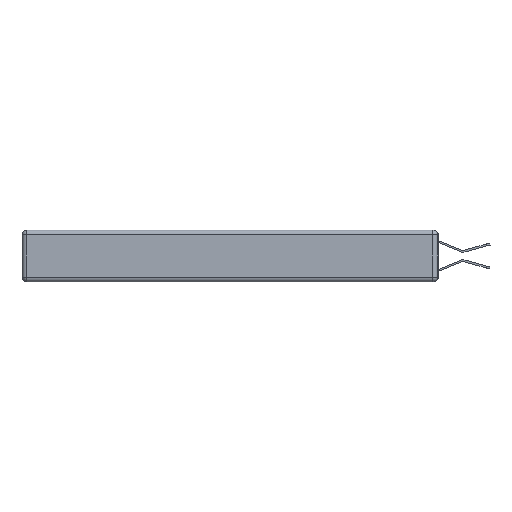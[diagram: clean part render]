
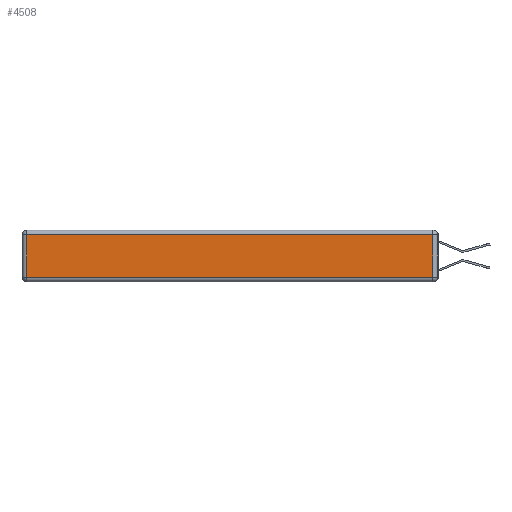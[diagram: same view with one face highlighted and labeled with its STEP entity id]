
A CAD part, left-side view. The second image highlights one B-rep face of the part: STEP entity #4508.
In plain terms, the highlighted planar face has unit normal (-1, 0, 0).
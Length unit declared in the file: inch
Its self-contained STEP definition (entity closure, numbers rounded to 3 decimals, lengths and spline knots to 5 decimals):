
#93 = DIRECTION ( 'NONE',  ( -1., 0., 0. ) ) ;
#626 = AXIS2_PLACEMENT_3D ( 'NONE', #4686, #93, #10742 ) ;
#983 = VECTOR ( 'NONE', #1084, 39.37008 ) ;
#1084 = DIRECTION ( 'NONE',  ( 0., 0., 1. ) ) ;
#1386 = CARTESIAN_POINT ( 'NONE',  ( 0., 2.72, -0.03 ) ) ;
#1850 = ORIENTED_EDGE ( 'NONE', *, *, #13331, .T. ) ;
#2027 = DIRECTION ( 'NONE',  ( 0., -1., 0. ) ) ;
#4492 = CARTESIAN_POINT ( 'NONE',  ( 0., 0., -0.313 ) ) ;
#4508 = ADVANCED_FACE ( 'NONE', ( #4921 ), #4766, .T. ) ;
#4585 = LINE ( 'NONE', #10493, #5303 ) ;
#4686 = CARTESIAN_POINT ( 'NONE',  ( 0., 0., -0.343 ) ) ;
#4766 = PLANE ( 'NONE',  #626 ) ;
#4921 = FACE_OUTER_BOUND ( 'NONE', #10962, .T. ) ;
#5303 = VECTOR ( 'NONE', #11910, 39.37008 ) ;
#7315 = CARTESIAN_POINT ( 'NONE',  ( 0., 0.03, -0.313 ) ) ;
#7919 = EDGE_CURVE ( 'NONE', #13001, #8813, #8820, .T. ) ;
#8742 = CARTESIAN_POINT ( 'NONE',  ( 0., 2.72, -0.313 ) ) ;
#8813 = VERTEX_POINT ( 'NONE', #1386 ) ;
#8820 = LINE ( 'NONE', #15041, #11105 ) ;
#9033 = VERTEX_POINT ( 'NONE', #8742 ) ;
#9103 = ORIENTED_EDGE ( 'NONE', *, *, #13421, .T. ) ;
#9520 = LINE ( 'NONE', #11983, #983 ) ;
#10493 = CARTESIAN_POINT ( 'NONE',  ( 0., 2.72, -0.343 ) ) ;
#10742 = DIRECTION ( 'NONE',  ( 0., 0., 1. ) ) ;
#10753 = ORIENTED_EDGE ( 'NONE', *, *, #13826, .T. ) ;
#10962 = EDGE_LOOP ( 'NONE', ( #10753, #9103, #13102, #1850 ) ) ;
#11105 = VECTOR ( 'NONE', #14879, 39.37008 ) ;
#11910 = DIRECTION ( 'NONE',  ( 0., 0., -1. ) ) ;
#11983 = CARTESIAN_POINT ( 'NONE',  ( 0., 0.03, -0.343 ) ) ;
#13001 = VERTEX_POINT ( 'NONE', #13452 ) ;
#13102 = ORIENTED_EDGE ( 'NONE', *, *, #7919, .T. ) ;
#13331 = EDGE_CURVE ( 'NONE', #8813, #9033, #4585, .T. ) ;
#13421 = EDGE_CURVE ( 'NONE', #15464, #13001, #9520, .T. ) ;
#13452 = CARTESIAN_POINT ( 'NONE',  ( 0., 0.03, -0.03 ) ) ;
#13826 = EDGE_CURVE ( 'NONE', #9033, #15464, #15497, .T. ) ;
#13974 = VECTOR ( 'NONE', #2027, 39.37008 ) ;
#14879 = DIRECTION ( 'NONE',  ( 0., 1., 0. ) ) ;
#15041 = CARTESIAN_POINT ( 'NONE',  ( 0., 2.75, -0.03 ) ) ;
#15464 = VERTEX_POINT ( 'NONE', #7315 ) ;
#15497 = LINE ( 'NONE', #4492, #13974 ) ;
